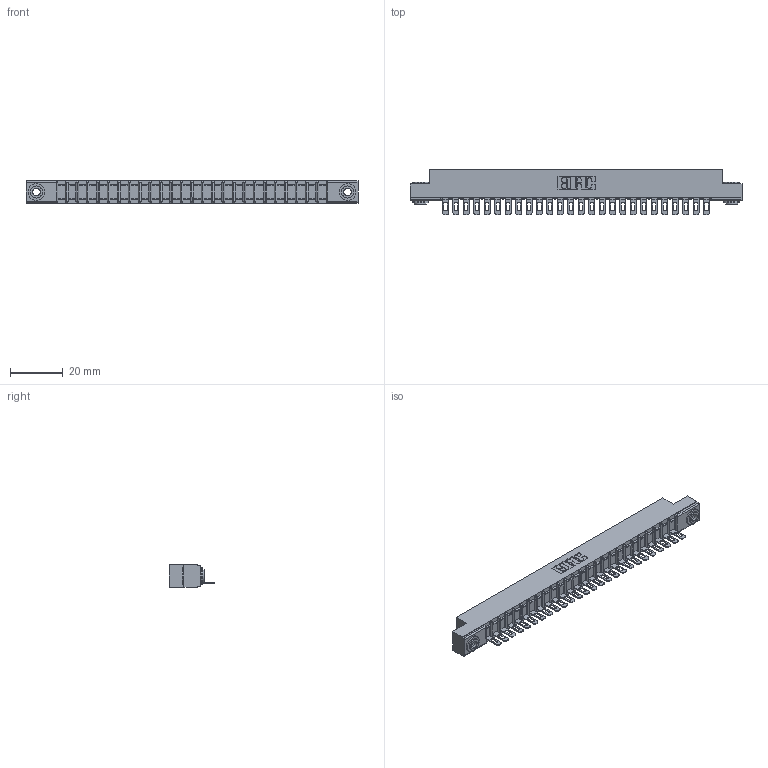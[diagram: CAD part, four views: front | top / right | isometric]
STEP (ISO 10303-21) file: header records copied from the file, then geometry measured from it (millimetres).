
FILE_DESCRIPTION (( 'STEP AP203' ), '1' );
FILE_NAME ('307-026-501-103.STEP', '2018-08-04T13:52:44', ( '' ), ( '' ), 'SwSTEP 2.0', 'SolidWorks 2016', '' );
FILE_SCHEMA (( 'CONFIG_CONTROL_DESIGN' ));
Length unit declared in the file: inch
Products named in the file (4): 307-026-501-103; 307 Part_.156 Dia Mounting Holes; 307-290-002_501; 345-250-002_345-250-002-102
Assembly tree (29 placements, depth 2):
  307-026-501-103
    307 Part_.156 Dia Mounting Holes
    307-290-002_501  x26
    345-250-002_345-250-002-102  x2
Bounding box: 126.03 x 17.42 x 8.71 mm (x, y, z)
Volume: 8346.6 mm3; surface area: 15822.5 mm2
Topology: 29 solids, 29 shells, 2173 faces, 6623 edges, 4338 vertices
Faces by surface type: plane 1238, cylinder 873, sphere 54, cone 8
Entity records: 26121 total; most frequent: CARTESIAN_POINT 4381, ORIENTED_EDGE 4362, DIRECTION 4283, EDGE_CURVE 2181, VECTOR 1651, LINE 1651, VERTEX_POINT 1414, AXIS2_PLACEMENT_3D 1316
